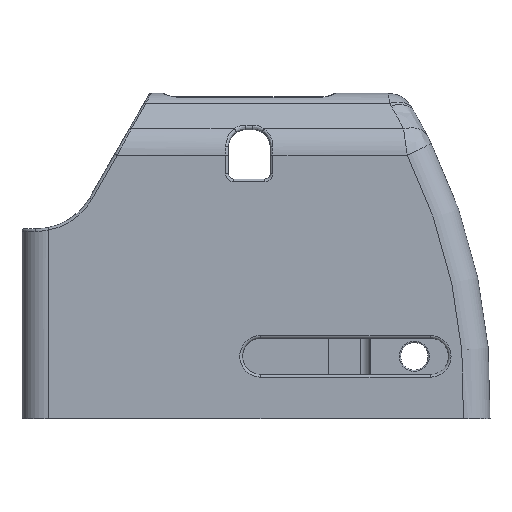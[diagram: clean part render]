
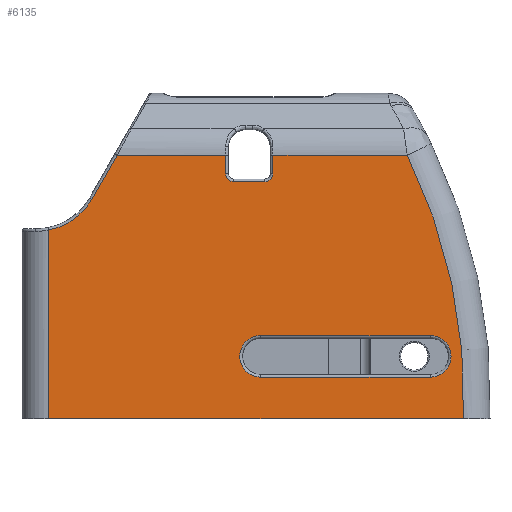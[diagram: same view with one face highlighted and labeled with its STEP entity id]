
A CAD part, left-side view. The second image highlights one B-rep face of the part: STEP entity #6135.
In plain terms, the highlighted planar face has unit normal (-1, 0, 0).
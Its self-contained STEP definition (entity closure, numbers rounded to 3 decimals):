
#345=FACE_BOUND('',#1933,.T.);
#403=PLANE('',#6759);
#702=LINE('',#12468,#1078);
#705=LINE('',#12483,#1081);
#713=LINE('',#12533,#1089);
#714=LINE('',#12537,#1090);
#715=LINE('',#12539,#1091);
#716=LINE('',#12543,#1092);
#717=LINE('',#12545,#1093);
#718=LINE('',#12549,#1094);
#719=LINE('',#12553,#1095);
#720=LINE('',#12554,#1096);
#1078=VECTOR('',#8153,10.);
#1081=VECTOR('',#8170,10.);
#1089=VECTOR('',#8198,10.);
#1090=VECTOR('',#8201,10.);
#1091=VECTOR('',#8202,10.);
#1092=VECTOR('',#8205,10.);
#1093=VECTOR('',#8206,10.);
#1094=VECTOR('',#8209,10.);
#1095=VECTOR('',#8212,10.);
#1096=VECTOR('',#8213,10.);
#1555=FACE_OUTER_BOUND('',#1932,.T.);
#1932=EDGE_LOOP('',(#5104,#5105,#5106,#5107,#5108,#5109,#5110,#5111,#5112,
#5113,#5114,#5115));
#1933=EDGE_LOOP('',(#5116,#5117,#5118,#5119));
#2312=CIRCLE('',#6747,3.925);
#2315=CIRCLE('',#6752,3.925);
#2320=CIRCLE('',#6760,12.);
#2321=CIRCLE('',#6761,103.5);
#2322=CIRCLE('',#6762,1.5);
#2323=CIRCLE('',#6763,1.5);
#2851=VERTEX_POINT('',#12465);
#2852=VERTEX_POINT('',#12467);
#2854=VERTEX_POINT('',#12473);
#2856=VERTEX_POINT('',#12479);
#2868=VERTEX_POINT('',#12531);
#2869=VERTEX_POINT('',#12532);
#2870=VERTEX_POINT('',#12534);
#2871=VERTEX_POINT('',#12536);
#2872=VERTEX_POINT('',#12538);
#2873=VERTEX_POINT('',#12540);
#2874=VERTEX_POINT('',#12542);
#2875=VERTEX_POINT('',#12544);
#2876=VERTEX_POINT('',#12546);
#2877=VERTEX_POINT('',#12548);
#2878=VERTEX_POINT('',#12550);
#2879=VERTEX_POINT('',#12552);
#3654=EDGE_CURVE('',#2851,#2852,#702,.T.);
#3659=EDGE_CURVE('',#2852,#2854,#2312,.T.);
#3662=EDGE_CURVE('',#2854,#2856,#705,.T.);
#3664=EDGE_CURVE('',#2856,#2851,#2315,.T.);
#3678=EDGE_CURVE('',#2868,#2869,#713,.T.);
#3679=EDGE_CURVE('',#2870,#2868,#2320,.T.);
#3680=EDGE_CURVE('',#2871,#2870,#714,.T.);
#3681=EDGE_CURVE('',#2871,#2872,#715,.F.);
#3682=EDGE_CURVE('',#2873,#2872,#2321,.T.);
#3683=EDGE_CURVE('',#2873,#2874,#716,.T.);
#3684=EDGE_CURVE('',#2875,#2874,#717,.T.);
#3685=EDGE_CURVE('',#2876,#2875,#2322,.T.);
#3686=EDGE_CURVE('',#2877,#2876,#718,.T.);
#3687=EDGE_CURVE('',#2878,#2877,#2323,.T.);
#3688=EDGE_CURVE('',#2879,#2878,#719,.T.);
#3689=EDGE_CURVE('',#2879,#2869,#720,.T.);
#5104=ORIENTED_EDGE('',*,*,#3678,.F.);
#5105=ORIENTED_EDGE('',*,*,#3679,.F.);
#5106=ORIENTED_EDGE('',*,*,#3680,.F.);
#5107=ORIENTED_EDGE('',*,*,#3681,.T.);
#5108=ORIENTED_EDGE('',*,*,#3682,.F.);
#5109=ORIENTED_EDGE('',*,*,#3683,.T.);
#5110=ORIENTED_EDGE('',*,*,#3684,.F.);
#5111=ORIENTED_EDGE('',*,*,#3685,.F.);
#5112=ORIENTED_EDGE('',*,*,#3686,.F.);
#5113=ORIENTED_EDGE('',*,*,#3687,.F.);
#5114=ORIENTED_EDGE('',*,*,#3688,.F.);
#5115=ORIENTED_EDGE('',*,*,#3689,.T.);
#5116=ORIENTED_EDGE('',*,*,#3654,.F.);
#5117=ORIENTED_EDGE('',*,*,#3664,.F.);
#5118=ORIENTED_EDGE('',*,*,#3662,.F.);
#5119=ORIENTED_EDGE('',*,*,#3659,.F.);
#6135=ADVANCED_FACE('',(#1555,#345),#403,.F.);
#6747=AXIS2_PLACEMENT_3D('',#12477,#8163,#8164);
#6752=AXIS2_PLACEMENT_3D('',#12486,#8175,#8176);
#6759=AXIS2_PLACEMENT_3D('',#12530,#8196,#8197);
#6760=AXIS2_PLACEMENT_3D('',#12535,#8199,#8200);
#6761=AXIS2_PLACEMENT_3D('',#12541,#8203,#8204);
#6762=AXIS2_PLACEMENT_3D('',#12547,#8207,#8208);
#6763=AXIS2_PLACEMENT_3D('',#12551,#8210,#8211);
#8153=DIRECTION('',(0.,-1.,0.));
#8163=DIRECTION('center_axis',(-1.,0.,0.));
#8164=DIRECTION('ref_axis',(0.,-1.,0.));
#8170=DIRECTION('',(0.,1.,0.));
#8175=DIRECTION('center_axis',(-1.,0.,0.));
#8176=DIRECTION('ref_axis',(0.,1.,0.));
#8196=DIRECTION('center_axis',(1.,0.,0.));
#8197=DIRECTION('ref_axis',(0.,0.,-1.));
#8198=DIRECTION('',(0.,-0.499,0.866));
#8199=DIRECTION('center_axis',(-1.,0.,0.));
#8200=DIRECTION('ref_axis',(0.,-0.583,-0.812));
#8201=DIRECTION('',(0.,0.,1.));
#8202=DIRECTION('',(0.,1.,0.));
#8203=DIRECTION('center_axis',(1.,0.,0.));
#8204=DIRECTION('ref_axis',(0.,-0.976,0.216));
#8205=DIRECTION('',(0.,1.,0.));
#8206=DIRECTION('',(0.,0.,1.));
#8207=DIRECTION('center_axis',(-1.,0.,0.));
#8208=DIRECTION('ref_axis',(0.,-0.707,-0.707));
#8209=DIRECTION('',(0.,-1.,0.));
#8210=DIRECTION('center_axis',(-1.,0.,0.));
#8211=DIRECTION('ref_axis',(0.,0.707,-0.707));
#8212=DIRECTION('',(0.,0.,-1.));
#8213=DIRECTION('',(0.,1.,0.));
#12465=CARTESIAN_POINT('',(-118.44,-13.233,-12.45));
#12467=CARTESIAN_POINT('',(-118.44,-45.212,-12.45));
#12468=CARTESIAN_POINT('',(-118.44,-12.819,-12.45));
#12473=CARTESIAN_POINT('',(-118.44,-45.212,-4.6));
#12477=CARTESIAN_POINT('Origin',(-118.44,-45.212,-8.525));
#12479=CARTESIAN_POINT('',(-118.44,-13.233,-4.6));
#12483=CARTESIAN_POINT('',(-118.44,-12.819,-4.6));
#12486=CARTESIAN_POINT('Origin',(-118.44,-13.233,-8.525));
#12530=CARTESIAN_POINT('Origin',(-118.44,-12.406,8.812));
#12531=CARTESIAN_POINT('',(-118.44,18.591,21.057));
#12532=CARTESIAN_POINT('',(-118.44,13.797,29.372));
#12533=CARTESIAN_POINT('',(-118.44,11.452,33.44));
#12534=CARTESIAN_POINT('',(-118.44,26.734,15.264));
#12535=CARTESIAN_POINT('Origin',(-118.44,28.987,27.051));
#12536=CARTESIAN_POINT('',(-118.44,26.734,-20.259));
#12537=CARTESIAN_POINT('',(-118.44,26.734,14.575));
#12538=CARTESIAN_POINT('',(-118.44,-51.472,-20.259));
#12539=CARTESIAN_POINT('',(-118.44,-6.203,-20.259));
#12540=CARTESIAN_POINT('',(-118.44,-40.894,29.372));
#12541=CARTESIAN_POINT('Origin',(-118.44,51.954,-16.36));
#12542=CARTESIAN_POINT('',(-118.44,-15.567,29.372));
#12543=CARTESIAN_POINT('',(-118.44,-56.546,29.372));
#12544=CARTESIAN_POINT('',(-118.44,-15.567,25.905));
#12545=CARTESIAN_POINT('',(-118.44,-15.567,16.859));
#12546=CARTESIAN_POINT('',(-118.44,-14.067,24.405));
#12547=CARTESIAN_POINT('Origin',(-118.44,-14.067,25.905));
#12548=CARTESIAN_POINT('',(-118.44,-8.167,24.405));
#12549=CARTESIAN_POINT('',(-118.44,-9.786,24.405));
#12550=CARTESIAN_POINT('',(-118.44,-6.667,25.905));
#12551=CARTESIAN_POINT('Origin',(-118.44,-8.167,25.905));
#12552=CARTESIAN_POINT('',(-118.44,-6.667,29.372));
#12553=CARTESIAN_POINT('',(-118.44,-6.667,19.859));
#12554=CARTESIAN_POINT('',(-118.44,-56.546,29.372));
